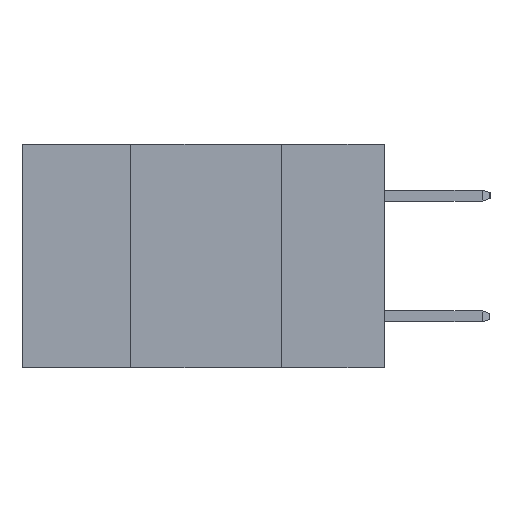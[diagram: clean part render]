
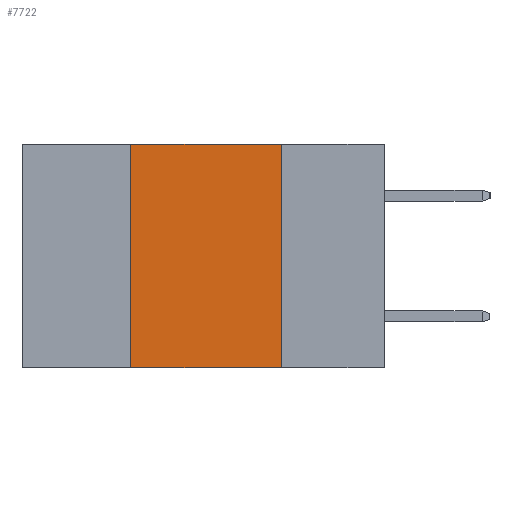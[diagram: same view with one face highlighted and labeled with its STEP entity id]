
A CAD part, left-side view. The second image highlights one B-rep face of the part: STEP entity #7722.
In plain terms, the highlighted planar face has unit normal (-1, 0, 0).
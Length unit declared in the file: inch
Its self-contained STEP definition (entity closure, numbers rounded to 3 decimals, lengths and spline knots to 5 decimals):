
#412 = VERTEX_POINT ( 'NONE', #3244 ) ;
#522 = DIRECTION ( 'NONE',  ( 0., -1., 0. ) ) ;
#1274 = ORIENTED_EDGE ( 'NONE', *, *, #4705, .T. ) ;
#1494 = VECTOR ( 'NONE', #522, 39.37008 ) ;
#1539 = CARTESIAN_POINT ( 'NONE',  ( 0., 0.17, 0. ) ) ;
#1897 = ORIENTED_EDGE ( 'NONE', *, *, #4176, .F. ) ;
#2009 = ORIENTED_EDGE ( 'NONE', *, *, #2498, .F. ) ;
#2072 = CARTESIAN_POINT ( 'NONE',  ( 0., 0.17, 0. ) ) ;
#2125 = LINE ( 'NONE', #4633, #10548 ) ;
#2284 = LINE ( 'NONE', #2072, #8588 ) ;
#2498 = EDGE_CURVE ( 'NONE', #6877, #7656, #2284, .T. ) ;
#2754 = DIRECTION ( 'NONE',  ( 0., -1., 0. ) ) ;
#3241 = EDGE_CURVE ( 'NONE', #10439, #6877, #2125, .T. ) ;
#3244 = CARTESIAN_POINT ( 'NONE',  ( 0., 0.42, -0.37 ) ) ;
#3899 = CARTESIAN_POINT ( 'NONE',  ( 0., 0.42, 0. ) ) ;
#4176 = EDGE_CURVE ( 'NONE', #412, #10439, #8936, .T. ) ;
#4568 = VECTOR ( 'NONE', #5489, 39.37008 ) ;
#4633 = CARTESIAN_POINT ( 'NONE',  ( 0., 0.6, 0. ) ) ;
#4705 = EDGE_CURVE ( 'NONE', #412, #7656, #5938, .T. ) ;
#5489 = DIRECTION ( 'NONE',  ( 0., 0., 1. ) ) ;
#5938 = LINE ( 'NONE', #7517, #1494 ) ;
#6324 = AXIS2_PLACEMENT_3D ( 'NONE', #8584, #8690, #8703 ) ;
#6793 = DIRECTION ( 'NONE',  ( 0., 0., -1. ) ) ;
#6877 = VERTEX_POINT ( 'NONE', #1539 ) ;
#6882 = CARTESIAN_POINT ( 'NONE',  ( 0., 0.17, -0.37 ) ) ;
#7243 = EDGE_LOOP ( 'NONE', ( #2009, #9429, #1897, #1274 ) ) ;
#7517 = CARTESIAN_POINT ( 'NONE',  ( 0., 0.6, -0.37 ) ) ;
#7656 = VERTEX_POINT ( 'NONE', #6882 ) ;
#7722 = ADVANCED_FACE ( 'NONE', ( #7773 ), #7924, .F. ) ;
#7773 = FACE_OUTER_BOUND ( 'NONE', #7243, .T. ) ;
#7924 = PLANE ( 'NONE',  #6324 ) ;
#8584 = CARTESIAN_POINT ( 'NONE',  ( 0., 0.6, 0. ) ) ;
#8588 = VECTOR ( 'NONE', #6793, 39.37008 ) ;
#8690 = DIRECTION ( 'NONE',  ( 1., 0., 0. ) ) ;
#8703 = DIRECTION ( 'NONE',  ( 0., 0., -1. ) ) ;
#8936 = LINE ( 'NONE', #9501, #4568 ) ;
#9429 = ORIENTED_EDGE ( 'NONE', *, *, #3241, .F. ) ;
#9501 = CARTESIAN_POINT ( 'NONE',  ( 0., 0.42, 0. ) ) ;
#10439 = VERTEX_POINT ( 'NONE', #3899 ) ;
#10548 = VECTOR ( 'NONE', #2754, 39.37008 ) ;
